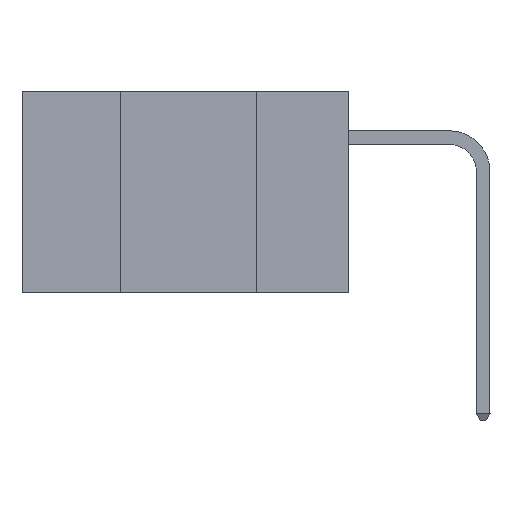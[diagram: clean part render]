
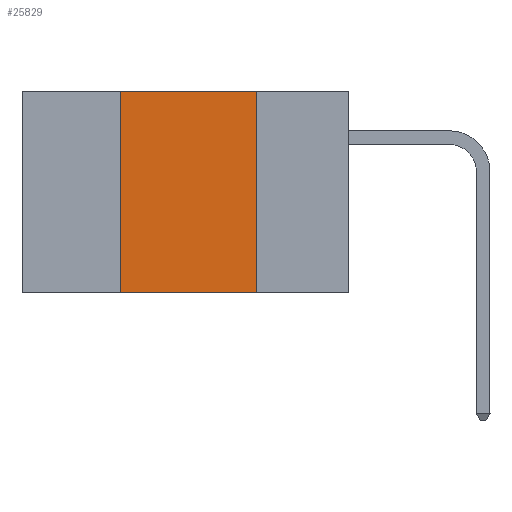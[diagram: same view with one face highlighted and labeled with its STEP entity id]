
A CAD part, left-side view. The second image highlights one B-rep face of the part: STEP entity #25829.
In plain terms, the highlighted planar face has unit normal (-1, 0, 0).
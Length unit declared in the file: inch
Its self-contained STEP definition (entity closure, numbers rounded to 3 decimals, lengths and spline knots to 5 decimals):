
#918 = EDGE_CURVE ( 'NONE', #8568, #7506, #2526, .T. ) ;
#1045 = CARTESIAN_POINT ( 'NONE',  ( 0., 0.6, 0. ) ) ;
#1441 = DIRECTION ( 'NONE',  ( 1., 0., 0. ) ) ;
#2116 = CARTESIAN_POINT ( 'NONE',  ( 0., 0.17, 0. ) ) ;
#2526 = LINE ( 'NONE', #1045, #9960 ) ;
#3892 = DIRECTION ( 'NONE',  ( 0., 0., -1. ) ) ;
#4779 = ORIENTED_EDGE ( 'NONE', *, *, #25498, .F. ) ;
#5760 = AXIS2_PLACEMENT_3D ( 'NONE', #18049, #1441, #11464 ) ;
#5919 = LINE ( 'NONE', #2116, #24234 ) ;
#6331 = DIRECTION ( 'NONE',  ( 0., 0., 1. ) ) ;
#7506 = VERTEX_POINT ( 'NONE', #22503 ) ;
#8184 = ORIENTED_EDGE ( 'NONE', *, *, #23009, .F. ) ;
#8568 = VERTEX_POINT ( 'NONE', #9820 ) ;
#8643 = CARTESIAN_POINT ( 'NONE',  ( 0., 0.17, -0.37 ) ) ;
#9287 = FACE_OUTER_BOUND ( 'NONE', #21365, .T. ) ;
#9820 = CARTESIAN_POINT ( 'NONE',  ( 0., 0.42, 0. ) ) ;
#9960 = VECTOR ( 'NONE', #11460, 39.37008 ) ;
#9980 = CARTESIAN_POINT ( 'NONE',  ( 0., 0.42, 0. ) ) ;
#10062 = VECTOR ( 'NONE', #6331, 39.37008 ) ;
#10524 = VECTOR ( 'NONE', #11952, 39.37008 ) ;
#11175 = CARTESIAN_POINT ( 'NONE',  ( 0., 0.42, -0.37 ) ) ;
#11460 = DIRECTION ( 'NONE',  ( 0., -1., 0. ) ) ;
#11464 = DIRECTION ( 'NONE',  ( 0., 0., -1. ) ) ;
#11952 = DIRECTION ( 'NONE',  ( 0., -1., 0. ) ) ;
#14167 = LINE ( 'NONE', #9980, #10062 ) ;
#16809 = ORIENTED_EDGE ( 'NONE', *, *, #26362, .T. ) ;
#18049 = CARTESIAN_POINT ( 'NONE',  ( 0., 0.6, 0. ) ) ;
#19488 = ORIENTED_EDGE ( 'NONE', *, *, #918, .F. ) ;
#21365 = EDGE_LOOP ( 'NONE', ( #8184, #19488, #4779, #16809 ) ) ;
#21977 = PLANE ( 'NONE',  #5760 ) ;
#22503 = CARTESIAN_POINT ( 'NONE',  ( 0., 0.17, 0. ) ) ;
#23009 = EDGE_CURVE ( 'NONE', #7506, #23982, #5919, .T. ) ;
#23982 = VERTEX_POINT ( 'NONE', #8643 ) ;
#24234 = VECTOR ( 'NONE', #3892, 39.37008 ) ;
#24474 = VERTEX_POINT ( 'NONE', #11175 ) ;
#24747 = CARTESIAN_POINT ( 'NONE',  ( 0., 0.6, -0.37 ) ) ;
#25498 = EDGE_CURVE ( 'NONE', #24474, #8568, #14167, .T. ) ;
#25829 = ADVANCED_FACE ( 'NONE', ( #9287 ), #21977, .F. ) ;
#26362 = EDGE_CURVE ( 'NONE', #24474, #23982, #26375, .T. ) ;
#26375 = LINE ( 'NONE', #24747, #10524 ) ;
